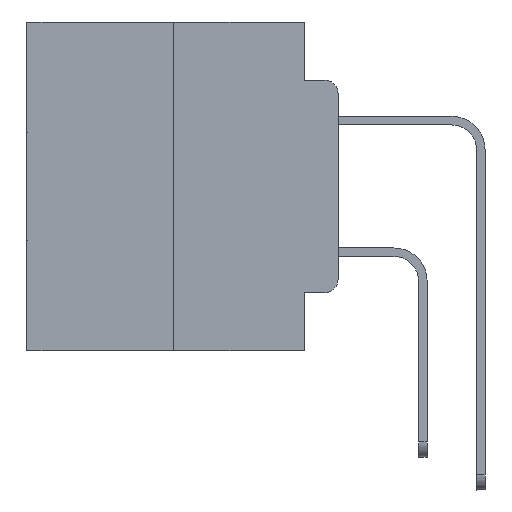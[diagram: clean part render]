
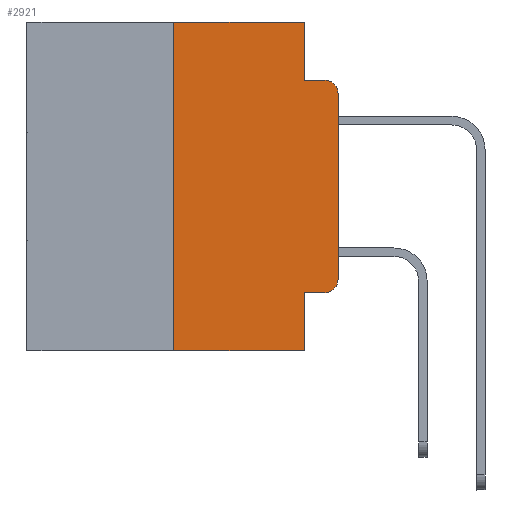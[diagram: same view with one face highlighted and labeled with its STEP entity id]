
A CAD part, left-side view. The second image highlights one B-rep face of the part: STEP entity #2921.
In plain terms, the highlighted planar face has unit normal (-1, 0, 0).
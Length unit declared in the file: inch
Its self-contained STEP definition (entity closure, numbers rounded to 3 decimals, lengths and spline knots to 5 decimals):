
#399 = EDGE_CURVE ( 'NONE', #15747, #15765, #10827, .T. ) ;
#1079 = CARTESIAN_POINT ( 'NONE',  ( 0., 0.02, -0.3915 ) ) ;
#1132 = ORIENTED_EDGE ( 'NONE', *, *, #399, .F. ) ;
#1461 = CARTESIAN_POINT ( 'NONE',  ( 0., 0., -0.1085 ) ) ;
#1635 = CARTESIAN_POINT ( 'NONE',  ( 0., 0., 0. ) ) ;
#2386 = CARTESIAN_POINT ( 'NONE',  ( 0., 0.051, 0. ) ) ;
#2508 = AXIS2_PLACEMENT_3D ( 'NONE', #26255, #11929, #28632 ) ;
#2636 = ORIENTED_EDGE ( 'NONE', *, *, #21945, .F. ) ;
#2921 = ADVANCED_FACE ( 'NONE', ( #6076 ), #9472, .F. ) ;
#3287 = CARTESIAN_POINT ( 'NONE',  ( 0., 0.051, -0.5 ) ) ;
#3541 = DIRECTION ( 'NONE',  ( 0., 0., -1. ) ) ;
#5249 = LINE ( 'NONE', #11153, #17374 ) ;
#6076 = FACE_OUTER_BOUND ( 'NONE', #25567, .T. ) ;
#6416 = VERTEX_POINT ( 'NONE', #13511 ) ;
#6486 = ORIENTED_EDGE ( 'NONE', *, *, #21998, .T. ) ;
#6843 = AXIS2_PLACEMENT_3D ( 'NONE', #1079, #18045, #3541 ) ;
#7564 = CARTESIAN_POINT ( 'NONE',  ( 0., 0.02, -0.0885 ) ) ;
#8582 = CARTESIAN_POINT ( 'NONE',  ( 0., 0.051, 0. ) ) ;
#8671 = CARTESIAN_POINT ( 'NONE',  ( 0., 0.051, -0.0885 ) ) ;
#8872 = VERTEX_POINT ( 'NONE', #18351 ) ;
#9087 = DIRECTION ( 'NONE',  ( 0., -1., 0. ) ) ;
#9472 = PLANE ( 'NONE',  #12312 ) ;
#9927 = LINE ( 'NONE', #1635, #15590 ) ;
#9980 = LINE ( 'NONE', #12481, #16403 ) ;
#10042 = VECTOR ( 'NONE', #9087, 39.37008 ) ;
#10425 = DIRECTION ( 'NONE',  ( 0., -1., 0. ) ) ;
#10702 = ORIENTED_EDGE ( 'NONE', *, *, #28060, .F. ) ;
#10827 = LINE ( 'NONE', #8671, #10042 ) ;
#11045 = DIRECTION ( 'NONE',  ( 0., 0., -1. ) ) ;
#11153 = CARTESIAN_POINT ( 'NONE',  ( 0., 0.473, -0.5 ) ) ;
#11468 = VECTOR ( 'NONE', #11045, 39.37008 ) ;
#11797 = ORIENTED_EDGE ( 'NONE', *, *, #21527, .T. ) ;
#11929 = DIRECTION ( 'NONE',  ( -1., 0., 0. ) ) ;
#12164 = LINE ( 'NONE', #27218, #29700 ) ;
#12312 = AXIS2_PLACEMENT_3D ( 'NONE', #30848, #28610, #14314 ) ;
#12481 = CARTESIAN_POINT ( 'NONE',  ( 0., 0.25, 0. ) ) ;
#12893 = DIRECTION ( 'NONE',  ( 0., -1., 0. ) ) ;
#12952 = LINE ( 'NONE', #8582, #11468 ) ;
#13014 = EDGE_CURVE ( 'NONE', #23323, #15765, #18951, .T. ) ;
#13511 = CARTESIAN_POINT ( 'NONE',  ( 0., 0.25, -0.5 ) ) ;
#13528 = VERTEX_POINT ( 'NONE', #18156 ) ;
#13554 = DIRECTION ( 'NONE',  ( 0., -1., 0. ) ) ;
#14314 = DIRECTION ( 'NONE',  ( 0., 0., -1. ) ) ;
#15560 = CIRCLE ( 'NONE', #6843, 0.02 ) ;
#15590 = VECTOR ( 'NONE', #16186, 39.37008 ) ;
#15747 = VERTEX_POINT ( 'NONE', #26667 ) ;
#15765 = VERTEX_POINT ( 'NONE', #7564 ) ;
#16186 = DIRECTION ( 'NONE',  ( 0., 0., 1. ) ) ;
#16403 = VECTOR ( 'NONE', #26803, 39.37008 ) ;
#16644 = VERTEX_POINT ( 'NONE', #27689 ) ;
#16777 = CARTESIAN_POINT ( 'NONE',  ( 0., 0., -0.3915 ) ) ;
#17050 = LINE ( 'NONE', #2386, #22674 ) ;
#17374 = VECTOR ( 'NONE', #13554, 39.37008 ) ;
#17839 = ORIENTED_EDGE ( 'NONE', *, *, #23821, .T. ) ;
#18045 = DIRECTION ( 'NONE',  ( -1., 0., 0. ) ) ;
#18156 = CARTESIAN_POINT ( 'NONE',  ( 0., 0.25, 0. ) ) ;
#18351 = CARTESIAN_POINT ( 'NONE',  ( 0., 0.02, -0.4115 ) ) ;
#18951 = CIRCLE ( 'NONE', #2508, 0.02 ) ;
#19342 = DIRECTION ( 'NONE',  ( 0., 0., -1. ) ) ;
#19498 = EDGE_CURVE ( 'NONE', #30595, #8872, #27294, .T. ) ;
#19698 = ORIENTED_EDGE ( 'NONE', *, *, #13014, .T. ) ;
#21436 = EDGE_CURVE ( 'NONE', #30595, #30970, #12952, .T. ) ;
#21527 = EDGE_CURVE ( 'NONE', #25328, #23323, #9927, .T. ) ;
#21945 = EDGE_CURVE ( 'NONE', #13528, #16644, #12164, .T. ) ;
#21998 = EDGE_CURVE ( 'NONE', #8872, #25328, #15560, .T. ) ;
#22674 = VECTOR ( 'NONE', #19342, 39.37008 ) ;
#23323 = VERTEX_POINT ( 'NONE', #1461 ) ;
#23821 = EDGE_CURVE ( 'NONE', #6416, #30970, #5249, .T. ) ;
#24156 = ORIENTED_EDGE ( 'NONE', *, *, #21436, .F. ) ;
#25328 = VERTEX_POINT ( 'NONE', #16777 ) ;
#25567 = EDGE_LOOP ( 'NONE', ( #11797, #19698, #1132, #27513, #2636, #10702, #17839, #24156, #30450, #6486 ) ) ;
#26255 = CARTESIAN_POINT ( 'NONE',  ( 0., 0.02, -0.1085 ) ) ;
#26537 = VECTOR ( 'NONE', #10425, 39.37008 ) ;
#26667 = CARTESIAN_POINT ( 'NONE',  ( 0., 0.051, -0.0885 ) ) ;
#26803 = DIRECTION ( 'NONE',  ( 0., 0., 1. ) ) ;
#27146 = CARTESIAN_POINT ( 'NONE',  ( 0., 0.051, -0.4115 ) ) ;
#27218 = CARTESIAN_POINT ( 'NONE',  ( 0., 0.473, 0. ) ) ;
#27294 = LINE ( 'NONE', #27146, #26537 ) ;
#27513 = ORIENTED_EDGE ( 'NONE', *, *, #29534, .F. ) ;
#27689 = CARTESIAN_POINT ( 'NONE',  ( 0., 0.051, 0. ) ) ;
#28060 = EDGE_CURVE ( 'NONE', #6416, #13528, #9980, .T. ) ;
#28610 = DIRECTION ( 'NONE',  ( 1., 0., 0. ) ) ;
#28632 = DIRECTION ( 'NONE',  ( 0., 0., -1. ) ) ;
#29534 = EDGE_CURVE ( 'NONE', #16644, #15747, #17050, .T. ) ;
#29700 = VECTOR ( 'NONE', #12893, 39.37008 ) ;
#30450 = ORIENTED_EDGE ( 'NONE', *, *, #19498, .T. ) ;
#30566 = CARTESIAN_POINT ( 'NONE',  ( 0., 0.051, -0.4115 ) ) ;
#30595 = VERTEX_POINT ( 'NONE', #30566 ) ;
#30848 = CARTESIAN_POINT ( 'NONE',  ( 0., 0.473, 0. ) ) ;
#30970 = VERTEX_POINT ( 'NONE', #3287 ) ;
